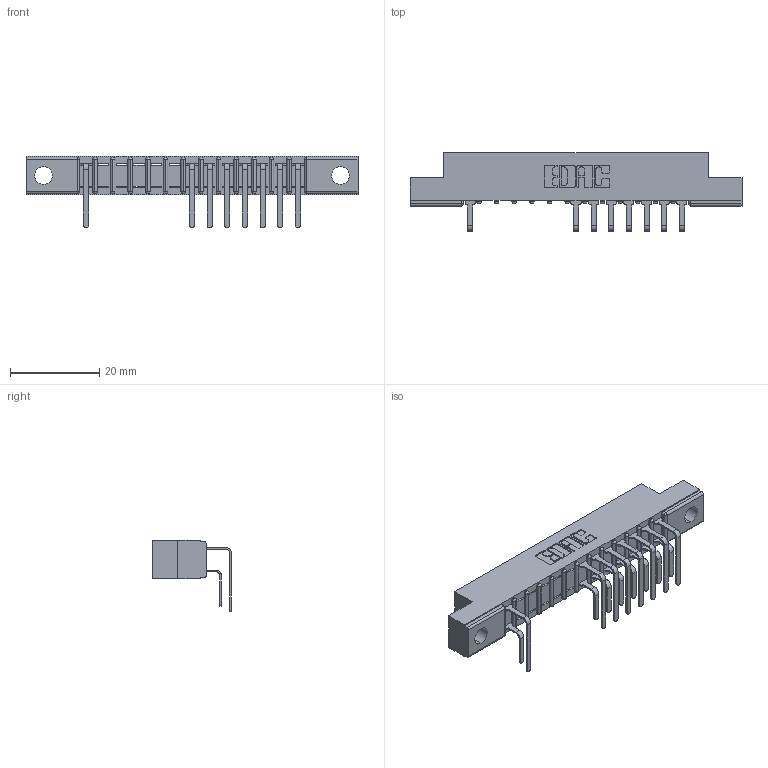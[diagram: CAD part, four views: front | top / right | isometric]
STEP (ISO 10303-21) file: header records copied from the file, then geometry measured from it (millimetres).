
FILE_DESCRIPTION (( 'STEP AP203' ), '1' );
FILE_NAME ('357-013-559-104.STEP', '2018-08-07T22:53:03', ( '' ), ( '' ), 'SwSTEP 2.0', 'SolidWorks 2016', '' );
FILE_SCHEMA (( 'CONFIG_CONTROL_DESIGN' ));
Length unit declared in the file: inch
Products named in the file (4): 307-290-001_559 - 2 (Single); 357-013-559-104; 307 Part_.156 Dia Mounting Holes; 307-290-001_558 559 - 1 (Single)
Assembly tree (17 placements, depth 2):
  357-013-559-104
    307 Part_.156 Dia Mounting Holes
    307-290-001_558 559 - 1 (Single)  x8
    307-290-001_559 - 2 (Single)  x8
Bounding box: 74.52 x 17.69 x 16.08 mm (x, y, z)
Volume: 4711.2 mm3; surface area: 7374.9 mm2
Topology: 17 solids, 17 shells, 1046 faces, 2951 edges, 1906 vertices
Faces by surface type: plane 672, cylinder 346, sphere 28
Entity records: 16681 total; most frequent: CARTESIAN_POINT 2787, ORIENTED_EDGE 2766, DIRECTION 2723, EDGE_CURVE 1383, VECTOR 1055, LINE 1055, VERTEX_POINT 898, AXIS2_PLACEMENT_3D 834
